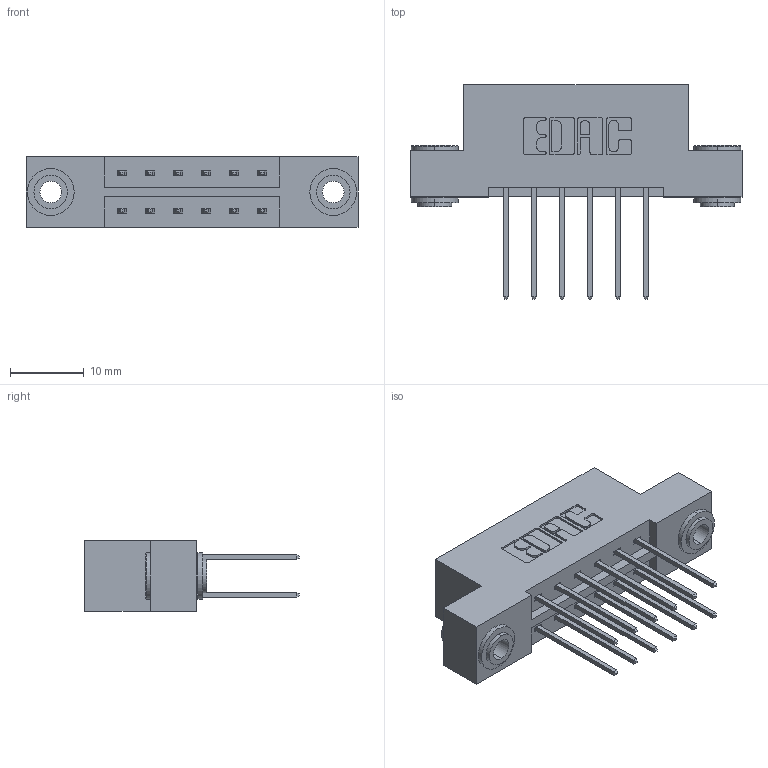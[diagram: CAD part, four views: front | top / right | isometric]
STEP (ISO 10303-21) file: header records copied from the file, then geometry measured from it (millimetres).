
FILE_DESCRIPTION (( 'STEP AP203' ), '1' );
FILE_NAME ('379-012-540-203.STEP', '2020-02-26T14:23:44', ( '' ), ( '' ), 'SwSTEP 2.0', 'SolidWorks 2016', '' );
FILE_SCHEMA (( 'CONFIG_CONTROL_DESIGN' ));
Length unit declared in the file: inch
Products named in the file (4): 345-292-001_345-293-140; 379-012-540-203; 379 Part_Flush - .156 Dia - TH; 345-250-002_345-250-002-102
Assembly tree (15 placements, depth 2):
  379-012-540-203
    379 Part_Flush - .156 Dia - TH
    345-292-001_345-293-140  x12
    345-250-002_345-250-002-102  x2
Bounding box: 45.09 x 29.13 x 9.53 mm (x, y, z)
Volume: 4412.6 mm3; surface area: 5074.4 mm2
Topology: 15 solids, 15 shells, 776 faces, 2247 edges, 1478 vertices
Faces by surface type: plane 512, cylinder 256, cone 8
Entity records: 9184 total; most frequent: CARTESIAN_POINT 1541, ORIENTED_EDGE 1470, DIRECTION 1413, EDGE_CURVE 735, LINE 583, VECTOR 583, VERTEX_POINT 486, AXIS2_PLACEMENT_3D 415
